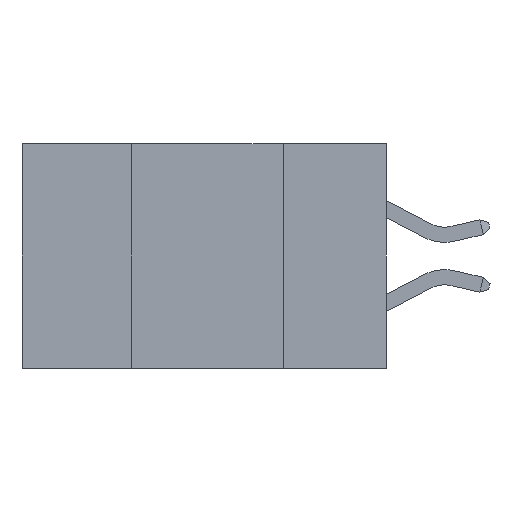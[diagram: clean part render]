
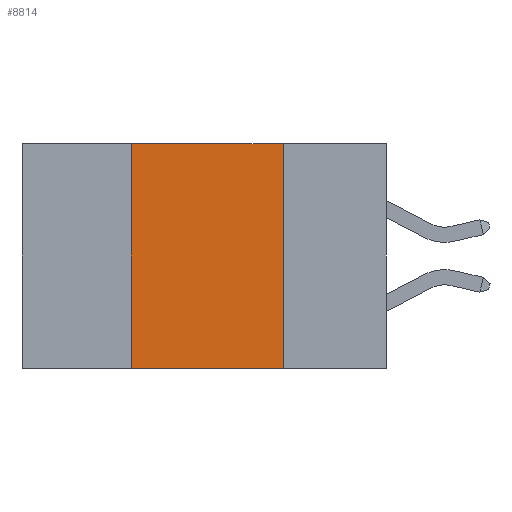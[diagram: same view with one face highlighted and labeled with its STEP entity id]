
A CAD part, left-side view. The second image highlights one B-rep face of the part: STEP entity #8814.
In plain terms, the highlighted planar face has unit normal (-1, 0, 0).
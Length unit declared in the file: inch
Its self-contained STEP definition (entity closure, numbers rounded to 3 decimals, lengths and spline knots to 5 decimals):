
#223 = AXIS2_PLACEMENT_3D ( 'NONE', #4045, #6315, #1392 ) ;
#247 = PLANE ( 'NONE',  #223 ) ;
#540 = CARTESIAN_POINT ( 'NONE',  ( 0., 0.42, 0. ) ) ;
#632 = EDGE_CURVE ( 'NONE', #3936, #9459, #6240, .T. ) ;
#639 = VECTOR ( 'NONE', #9066, 39.37008 ) ;
#662 = EDGE_CURVE ( 'NONE', #1696, #3936, #3496, .T. ) ;
#677 = EDGE_CURVE ( 'NONE', #1586, #1696, #3008, .T. ) ;
#678 = EDGE_CURVE ( 'NONE', #1586, #9459, #5055, .T. ) ;
#1247 = ORIENTED_EDGE ( 'NONE', *, *, #662, .F. ) ;
#1392 = DIRECTION ( 'NONE',  ( 0., 0., -1. ) ) ;
#1586 = VERTEX_POINT ( 'NONE', #2648 ) ;
#1696 = VERTEX_POINT ( 'NONE', #540 ) ;
#2648 = CARTESIAN_POINT ( 'NONE',  ( 0., 0.42, -0.37 ) ) ;
#3008 = LINE ( 'NONE', #9139, #639 ) ;
#3496 = LINE ( 'NONE', #10102, #7485 ) ;
#3936 = VERTEX_POINT ( 'NONE', #9550 ) ;
#4045 = CARTESIAN_POINT ( 'NONE',  ( 0., 0.6, 0. ) ) ;
#4727 = VECTOR ( 'NONE', #5426, 39.37008 ) ;
#5055 = LINE ( 'NONE', #9296, #8772 ) ;
#5426 = DIRECTION ( 'NONE',  ( 0., 0., -1. ) ) ;
#5446 = CARTESIAN_POINT ( 'NONE',  ( 0., 0.17, -0.37 ) ) ;
#5794 = CARTESIAN_POINT ( 'NONE',  ( 0., 0.17, -0.37 ) ) ;
#6240 = LINE ( 'NONE', #5446, #4727 ) ;
#6315 = DIRECTION ( 'NONE',  ( 1., 0., 0. ) ) ;
#7180 = EDGE_LOOP ( 'NONE', ( #9424, #1247, #7667, #9669 ) ) ;
#7485 = VECTOR ( 'NONE', #9785, 39.37008 ) ;
#7667 = ORIENTED_EDGE ( 'NONE', *, *, #677, .F. ) ;
#8772 = VECTOR ( 'NONE', #9171, 39.37008 ) ;
#8814 = ADVANCED_FACE ( 'NONE', ( #9287 ), #247, .F. ) ;
#9066 = DIRECTION ( 'NONE',  ( 0., 0., 1. ) ) ;
#9139 = CARTESIAN_POINT ( 'NONE',  ( 0., 0.42, -0.37 ) ) ;
#9171 = DIRECTION ( 'NONE',  ( 0., -1., 0. ) ) ;
#9287 = FACE_OUTER_BOUND ( 'NONE', #7180, .T. ) ;
#9296 = CARTESIAN_POINT ( 'NONE',  ( 0., 0.6, -0.37 ) ) ;
#9424 = ORIENTED_EDGE ( 'NONE', *, *, #632, .F. ) ;
#9459 = VERTEX_POINT ( 'NONE', #5794 ) ;
#9550 = CARTESIAN_POINT ( 'NONE',  ( 0., 0.17, 0. ) ) ;
#9669 = ORIENTED_EDGE ( 'NONE', *, *, #678, .T. ) ;
#9785 = DIRECTION ( 'NONE',  ( 0., -1., 0. ) ) ;
#10102 = CARTESIAN_POINT ( 'NONE',  ( 0., 0.6, 0. ) ) ;
